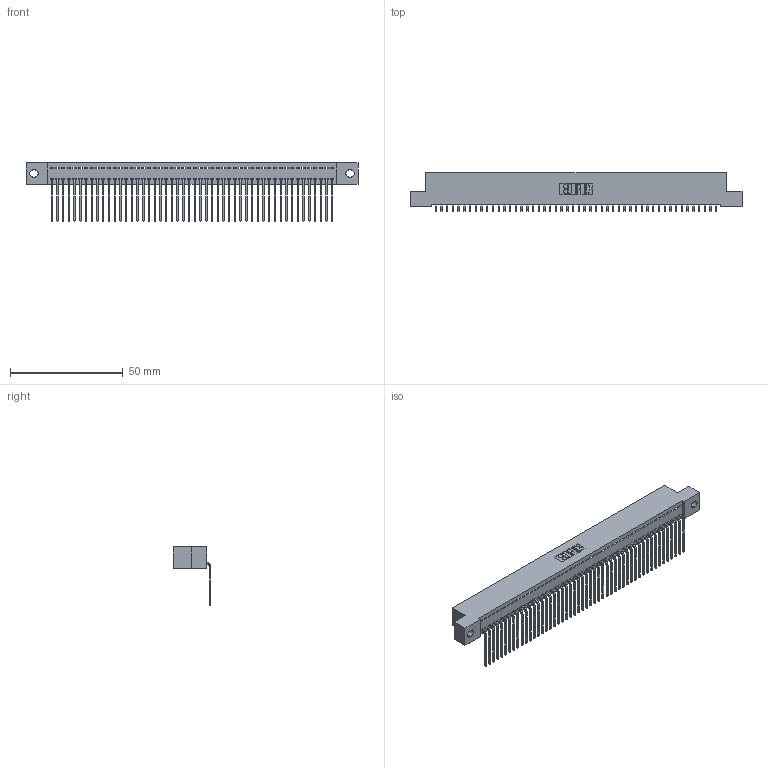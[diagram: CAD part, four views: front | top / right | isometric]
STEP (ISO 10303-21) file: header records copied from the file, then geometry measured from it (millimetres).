
FILE_DESCRIPTION (( 'STEP AP203' ), '1' );
FILE_NAME ('342-050-559-102.STEP', '2019-10-03T00:06:41', ( '' ), ( '' ), 'SwSTEP 2.0', 'SolidWorks 2016', '' );
FILE_SCHEMA (( 'CONFIG_CONTROL_DESIGN' ));
Length unit declared in the file: inch
Products named in the file (3): 342 Part_.128 Slot; 345-292-001_558 559 Tail - 1; 342-050-559-102
Assembly tree (51 placements, depth 2):
  342-050-559-102
    342 Part_.128 Slot
    345-292-001_558 559 Tail - 1  x50
Bounding box: 147.32 x 16.83 x 25.78 mm (x, y, z)
Volume: 13060.9 mm3; surface area: 20034.5 mm2
Topology: 51 solids, 51 shells, 3114 faces, 9411 edges, 6206 vertices
Faces by surface type: plane 2270, cylinder 844
Entity records: 29619 total; most frequent: CARTESIAN_POINT 5116, ORIENTED_EDGE 5102, DIRECTION 4299, EDGE_CURVE 2551, VECTOR 2423, LINE 2423, VERTEX_POINT 1698, AXIS2_PLACEMENT_3D 938
